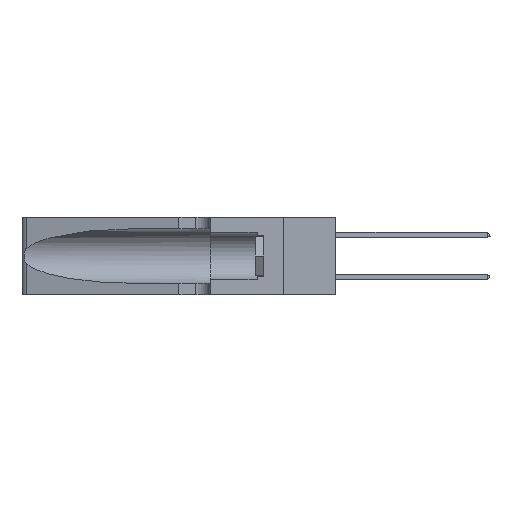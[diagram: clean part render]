
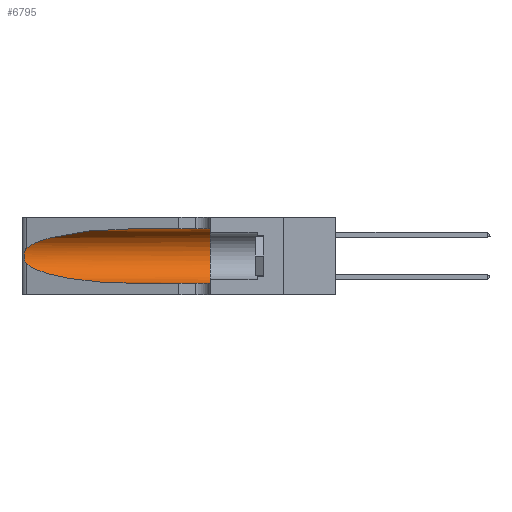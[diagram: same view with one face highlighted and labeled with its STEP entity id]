
A CAD part, left-side view. The second image highlights one B-rep face of the part: STEP entity #6795.
In plain terms, the highlighted cylindrical face has radius 3.308 mm (diameter 6.617 mm), a partial arc.
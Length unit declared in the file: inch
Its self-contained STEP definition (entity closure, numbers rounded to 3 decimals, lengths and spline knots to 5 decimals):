
#503 = ORIENTED_EDGE ( 'NONE', *, *, #4525, .T. ) ;
#559 = VERTEX_POINT ( 'NONE', #4425 ) ;
#701 = CARTESIAN_POINT ( 'NONE',  ( 0.25487, 1.22718, 0.14631 ) ) ;
#773 = CARTESIAN_POINT ( 'NONE',  ( 0.1305, 0.72297, 0.31525 ) ) ;
#1662 = LINE ( 'NONE', #5405, #10604 ) ;
#2228 = CARTESIAN_POINT ( 'NONE',  ( 0.1305, 0.72297, 0.05475 ) ) ;
#2534 = CARTESIAN_POINT ( 'NONE',  ( 0.18966, 0.96281, 0.05475 ) ) ;
#2643 =( BOUNDED_CURVE ( )  B_SPLINE_CURVE ( 3, ( #13809, #19197, #2670, #17789 ),
 .UNSPECIFIED., .F., .T. ) 
 B_SPLINE_CURVE_WITH_KNOTS ( ( 4, 4 ),
 ( 1.5708, 2.84003 ),
 .UNSPECIFIED. ) 
 CURVE ( )  GEOMETRIC_REPRESENTATION_ITEM ( )  RATIONAL_B_SPLINE_CURVE ( ( 1., 0.87, 0.87, 1. ) ) 
 REPRESENTATION_ITEM ( '' )  );
#2670 = CARTESIAN_POINT ( 'NONE',  ( 0.2373, 1.15595, 0.28018 ) ) ;
#3241 = AXIS2_PLACEMENT_3D ( 'NONE', #17707, #8065, #9992 ) ;
#3274 = CARTESIAN_POINT ( 'NONE',  ( 0.25487, 1.22718, 0.14631 ) ) ;
#3410 = ORIENTED_EDGE ( 'NONE', *, *, #15671, .T. ) ;
#3945 = DIRECTION ( 'NONE',  ( 0., -1., 0. ) ) ;
#4329 = EDGE_CURVE ( 'NONE', #7329, #8274, #16952, .T. ) ;
#4425 = CARTESIAN_POINT ( 'NONE',  ( 0.1305, 0.35, 0.05475 ) ) ;
#4525 = EDGE_CURVE ( 'NONE', #8274, #559, #1662, .T. ) ;
#4658 = CARTESIAN_POINT ( 'NONE',  ( 0.25854, 1.2359, 0.20912 ) ) ;
#4796 = CYLINDRICAL_SURFACE ( 'NONE', #6022, 0.13025 ) ;
#5177 = DIRECTION ( 'NONE',  ( 0., -1., 0. ) ) ;
#5405 = CARTESIAN_POINT ( 'NONE',  ( 0.1305, 1.61858, 0.05475 ) ) ;
#6022 = AXIS2_PLACEMENT_3D ( 'NONE', #7927, #3945, #6080 ) ;
#6080 = DIRECTION ( 'NONE',  ( 0., 0., -1. ) ) ;
#6484 = CARTESIAN_POINT ( 'NONE',  ( 0.25487, 1.22718, 0.22369 ) ) ;
#6511 = CARTESIAN_POINT ( 'NONE',  ( 0.2373, 1.15595, 0.08982 ) ) ;
#6565 = CARTESIAN_POINT ( 'NONE',  ( 0.26075, 1.23896, 0.19203 ) ) ;
#6645 = CARTESIAN_POINT ( 'NONE',  ( 0.25639, 1.23186, 0.15144 ) ) ;
#6795 = ADVANCED_FACE ( 'NONE', ( #12552 ), #4796, .F. ) ;
#6971 = VERTEX_POINT ( 'NONE', #773 ) ;
#7018 = EDGE_LOOP ( 'NONE', ( #19565, #3410, #15807, #503, #13228, #8441 ) ) ;
#7329 = VERTEX_POINT ( 'NONE', #3274 ) ;
#7927 = CARTESIAN_POINT ( 'NONE',  ( 0.1305, 1.61858, 0.185 ) ) ;
#8065 = DIRECTION ( 'NONE',  ( 0., 1., 0. ) ) ;
#8274 = VERTEX_POINT ( 'NONE', #2228 ) ;
#8320 = CARTESIAN_POINT ( 'NONE',  ( 0.26018, 1.23835, 0.19895 ) ) ;
#8441 = ORIENTED_EDGE ( 'NONE', *, *, #16716, .F. ) ;
#8696 = CARTESIAN_POINT ( 'NONE',  ( 0.25487, 1.22718, 0.22369 ) ) ;
#9547 = EDGE_CURVE ( 'NONE', #6971, #18506, #2643, .T. ) ;
#9992 = DIRECTION ( 'NONE',  ( 0., 0., 1. ) ) ;
#10421 = CARTESIAN_POINT ( 'NONE',  ( 0.25555, 1.22994, 0.2215 ) ) ;
#10449 = CARTESIAN_POINT ( 'NONE',  ( 0.1305, 0.72297, 0.05475 ) ) ;
#10604 = VECTOR ( 'NONE', #5177, 39.37008 ) ;
#10695 = VECTOR ( 'NONE', #20472, 39.37008 ) ;
#12325 = CARTESIAN_POINT ( 'NONE',  ( 0.25856, 1.23593, 0.16098 ) ) ;
#12552 = FACE_OUTER_BOUND ( 'NONE', #7018, .T. ) ;
#12643 = CARTESIAN_POINT ( 'NONE',  ( 0.25487, 1.22718, 0.14631 ) ) ;
#13228 = ORIENTED_EDGE ( 'NONE', *, *, #18856, .F. ) ;
#13264 = CARTESIAN_POINT ( 'NONE',  ( 0.1305, 0.35, 0.31525 ) ) ;
#13542 = CIRCLE ( 'NONE', #3241, 0.13025 ) ;
#13809 = CARTESIAN_POINT ( 'NONE',  ( 0.1305, 0.72297, 0.31525 ) ) ;
#15671 = EDGE_CURVE ( 'NONE', #18506, #7329, #21791, .T. ) ;
#15807 = ORIENTED_EDGE ( 'NONE', *, *, #4329, .T. ) ;
#16255 = CARTESIAN_POINT ( 'NONE',  ( 0.1305, 1.61858, 0.31525 ) ) ;
#16716 = EDGE_CURVE ( 'NONE', #6971, #23777, #21648, .T. ) ;
#16952 =( BOUNDED_CURVE ( )  B_SPLINE_CURVE ( 3, ( #701, #6511, #2534, #10449 ),
 .UNSPECIFIED., .F., .F. ) 
 B_SPLINE_CURVE_WITH_KNOTS ( ( 4, 4 ),
 ( 3.44316, 4.71239 ),
 .UNSPECIFIED. ) 
 CURVE ( )  GEOMETRIC_REPRESENTATION_ITEM ( )  RATIONAL_B_SPLINE_CURVE ( ( 1., 0.87, 0.87, 1. ) ) 
 REPRESENTATION_ITEM ( '' )  );
#17707 = CARTESIAN_POINT ( 'NONE',  ( 0.1305, 0.35, 0.185 ) ) ;
#17789 = CARTESIAN_POINT ( 'NONE',  ( 0.25487, 1.22718, 0.22369 ) ) ;
#18039 = CARTESIAN_POINT ( 'NONE',  ( 0.25789, 1.23486, 0.15765 ) ) ;
#18506 = VERTEX_POINT ( 'NONE', #8696 ) ;
#18856 = EDGE_CURVE ( 'NONE', #23777, #559, #13542, .T. ) ;
#19197 = CARTESIAN_POINT ( 'NONE',  ( 0.18966, 0.96281, 0.31525 ) ) ;
#19565 = ORIENTED_EDGE ( 'NONE', *, *, #9547, .T. ) ;
#19688 = CARTESIAN_POINT ( 'NONE',  ( 0.25787, 1.23484, 0.2124 ) ) ;
#19926 = CARTESIAN_POINT ( 'NONE',  ( 0.25555, 1.22993, 0.14849 ) ) ;
#20472 = DIRECTION ( 'NONE',  ( 0., -1., 0. ) ) ;
#21579 = CARTESIAN_POINT ( 'NONE',  ( 0.26075, 1.23896, 0.178 ) ) ;
#21648 = LINE ( 'NONE', #16255, #10695 ) ;
#21791 = B_SPLINE_CURVE_WITH_KNOTS ( 'NONE', 3,
 ( #6484, #10421, #23542, #19688, #4658, #8320, #6565, #21579, #23623, #12325, #18039, #6645, #19926, #12643 ),
 .UNSPECIFIED., .F., .F.,
 ( 4, 2, 2, 2, 2, 2, 4 ),
 ( 0., 0.00027, 0.00053, 0.00107, 0.0016, 0.00187, 0.00214 ),
 .UNSPECIFIED. ) ;
#23542 = CARTESIAN_POINT ( 'NONE',  ( 0.25639, 1.23184, 0.21858 ) ) ;
#23623 = CARTESIAN_POINT ( 'NONE',  ( 0.26017, 1.23833, 0.17102 ) ) ;
#23777 = VERTEX_POINT ( 'NONE', #13264 ) ;
